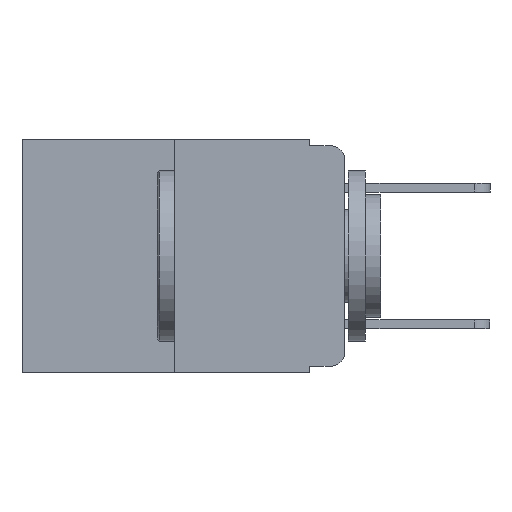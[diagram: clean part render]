
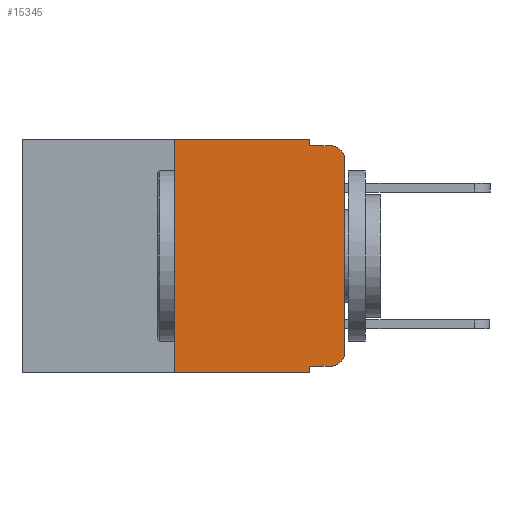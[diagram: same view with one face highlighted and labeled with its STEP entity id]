
A CAD part, left-side view. The second image highlights one B-rep face of the part: STEP entity #15345.
In plain terms, the highlighted planar face has unit normal (-1, 0, 0).
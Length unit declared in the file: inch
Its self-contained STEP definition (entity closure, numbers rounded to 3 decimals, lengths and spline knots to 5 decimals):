
#378 = ORIENTED_EDGE ( 'NONE', *, *, #2775, .F. ) ;
#384 = LINE ( 'NONE', #5873, #10076 ) ;
#818 = AXIS2_PLACEMENT_3D ( 'NONE', #1891, #3863, #16612 ) ;
#1452 = CARTESIAN_POINT ( 'NONE',  ( 0., 0.473, -0.343 ) ) ;
#1768 = DIRECTION ( 'NONE',  ( 0., 0., -1. ) ) ;
#1891 = CARTESIAN_POINT ( 'NONE',  ( 0., 0.473, 0. ) ) ;
#1912 = CARTESIAN_POINT ( 'NONE',  ( 0., 0.473, 0. ) ) ;
#1938 = LINE ( 'NONE', #1912, #16084 ) ;
#2481 = ORIENTED_EDGE ( 'NONE', *, *, #2853, .T. ) ;
#2502 = EDGE_CURVE ( 'NONE', #7574, #10900, #9524, .T. ) ;
#2510 = EDGE_CURVE ( 'NONE', #10900, #22518, #8947, .T. ) ;
#2661 = EDGE_CURVE ( 'NONE', #10622, #22518, #5360, .T. ) ;
#2775 = EDGE_CURVE ( 'NONE', #8996, #10622, #21219, .T. ) ;
#2814 = EDGE_CURVE ( 'NONE', #3269, #9903, #11227, .T. ) ;
#2821 = EDGE_CURVE ( 'NONE', #9942, #17237, #384, .T. ) ;
#2853 = EDGE_CURVE ( 'NONE', #9942, #9616, #18708, .T. ) ;
#2970 = EDGE_CURVE ( 'NONE', #9616, #7574, #5936, .T. ) ;
#3168 = CARTESIAN_POINT ( 'NONE',  ( 0., 0.051, -0.01 ) ) ;
#3269 = VERTEX_POINT ( 'NONE', #11419 ) ;
#3277 = EDGE_CURVE ( 'NONE', #9903, #8996, #1938, .T. ) ;
#3425 = ORIENTED_EDGE ( 'NONE', *, *, #2821, .F. ) ;
#3863 = DIRECTION ( 'NONE',  ( 1., 0., 0. ) ) ;
#4077 = DIRECTION ( 'NONE',  ( 0., -1., 0. ) ) ;
#4123 = ORIENTED_EDGE ( 'NONE', *, *, #3277, .F. ) ;
#4757 = VECTOR ( 'NONE', #17681, 39.37008 ) ;
#5012 = ORIENTED_EDGE ( 'NONE', *, *, #2510, .T. ) ;
#5159 = CARTESIAN_POINT ( 'NONE',  ( 0., 0.02, -0.01 ) ) ;
#5360 = LINE ( 'NONE', #3168, #4757 ) ;
#5873 = CARTESIAN_POINT ( 'NONE',  ( 0., 0.051, 0. ) ) ;
#5936 = CIRCLE ( 'NONE', #11740, 0.02 ) ;
#6531 = CARTESIAN_POINT ( 'NONE',  ( 0., 0., 0. ) ) ;
#6622 = CARTESIAN_POINT ( 'NONE',  ( 0., 0.02, -0.03 ) ) ;
#6682 = CARTESIAN_POINT ( 'NONE',  ( 0., 0.02, -0.313 ) ) ;
#6955 = AXIS2_PLACEMENT_3D ( 'NONE', #6622, #18895, #8502 ) ;
#7396 = DIRECTION ( 'NONE',  ( 0., -1., 0. ) ) ;
#7574 = VERTEX_POINT ( 'NONE', #7729 ) ;
#7729 = CARTESIAN_POINT ( 'NONE',  ( 0., 0., -0.313 ) ) ;
#8502 = DIRECTION ( 'NONE',  ( 0., 0., -1. ) ) ;
#8553 = DIRECTION ( 'NONE',  ( 0., 0., -1. ) ) ;
#8656 = CARTESIAN_POINT ( 'NONE',  ( 0., 0., -0.03 ) ) ;
#8947 = CIRCLE ( 'NONE', #6955, 0.02 ) ;
#8996 = VERTEX_POINT ( 'NONE', #12843 ) ;
#9441 = CARTESIAN_POINT ( 'NONE',  ( 0., 0.051, 0. ) ) ;
#9524 = LINE ( 'NONE', #6531, #17704 ) ;
#9616 = VERTEX_POINT ( 'NONE', #20699 ) ;
#9903 = VERTEX_POINT ( 'NONE', #11166 ) ;
#9942 = VERTEX_POINT ( 'NONE', #22882 ) ;
#10076 = VECTOR ( 'NONE', #18321, 39.37008 ) ;
#10622 = VERTEX_POINT ( 'NONE', #11567 ) ;
#10653 = ORIENTED_EDGE ( 'NONE', *, *, #2814, .F. ) ;
#10900 = VERTEX_POINT ( 'NONE', #8656 ) ;
#11166 = CARTESIAN_POINT ( 'NONE',  ( 0., 0.25, 0. ) ) ;
#11227 = LINE ( 'NONE', #16650, #19209 ) ;
#11419 = CARTESIAN_POINT ( 'NONE',  ( 0., 0.25, -0.343 ) ) ;
#11567 = CARTESIAN_POINT ( 'NONE',  ( 0., 0.051, -0.01 ) ) ;
#11740 = AXIS2_PLACEMENT_3D ( 'NONE', #6682, #18945, #8553 ) ;
#12324 = CARTESIAN_POINT ( 'NONE',  ( 0., 0.051, -0.343 ) ) ;
#12843 = CARTESIAN_POINT ( 'NONE',  ( 0., 0.051, 0. ) ) ;
#13165 = ORIENTED_EDGE ( 'NONE', *, *, #2661, .F. ) ;
#13184 = PLANE ( 'NONE',  #818 ) ;
#13389 = CARTESIAN_POINT ( 'NONE',  ( 0., 0.051, -0.333 ) ) ;
#13894 = LINE ( 'NONE', #1452, #22597 ) ;
#14418 = ORIENTED_EDGE ( 'NONE', *, *, #20543, .T. ) ;
#14885 = DIRECTION ( 'NONE',  ( 0., -1., 0. ) ) ;
#15345 = ADVANCED_FACE ( 'NONE', ( #15509 ), #13184, .F. ) ;
#15509 = FACE_OUTER_BOUND ( 'NONE', #21625, .T. ) ;
#15787 = ORIENTED_EDGE ( 'NONE', *, *, #2970, .T. ) ;
#15849 = VECTOR ( 'NONE', #1768, 39.37008 ) ;
#16084 = VECTOR ( 'NONE', #14885, 39.37008 ) ;
#16612 = DIRECTION ( 'NONE',  ( 0., 0., -1. ) ) ;
#16650 = CARTESIAN_POINT ( 'NONE',  ( 0., 0.25, 0. ) ) ;
#17237 = VERTEX_POINT ( 'NONE', #12324 ) ;
#17681 = DIRECTION ( 'NONE',  ( 0., -1., 0. ) ) ;
#17704 = VECTOR ( 'NONE', #20456, 39.37008 ) ;
#18200 = VECTOR ( 'NONE', #4077, 39.37008 ) ;
#18321 = DIRECTION ( 'NONE',  ( 0., 0., -1. ) ) ;
#18708 = LINE ( 'NONE', #13389, #18200 ) ;
#18895 = DIRECTION ( 'NONE',  ( -1., 0., 0. ) ) ;
#18945 = DIRECTION ( 'NONE',  ( -1., 0., 0. ) ) ;
#19209 = VECTOR ( 'NONE', #22987, 39.37008 ) ;
#20456 = DIRECTION ( 'NONE',  ( 0., 0., 1. ) ) ;
#20543 = EDGE_CURVE ( 'NONE', #3269, #17237, #13894, .T. ) ;
#20699 = CARTESIAN_POINT ( 'NONE',  ( 0., 0.02, -0.333 ) ) ;
#21119 = ORIENTED_EDGE ( 'NONE', *, *, #2502, .T. ) ;
#21219 = LINE ( 'NONE', #9441, #15849 ) ;
#21625 = EDGE_LOOP ( 'NONE', ( #21119, #5012, #13165, #378, #4123, #10653, #14418, #3425, #2481, #15787 ) ) ;
#22518 = VERTEX_POINT ( 'NONE', #5159 ) ;
#22597 = VECTOR ( 'NONE', #7396, 39.37008 ) ;
#22882 = CARTESIAN_POINT ( 'NONE',  ( 0., 0.051, -0.333 ) ) ;
#22987 = DIRECTION ( 'NONE',  ( 0., 0., 1. ) ) ;
